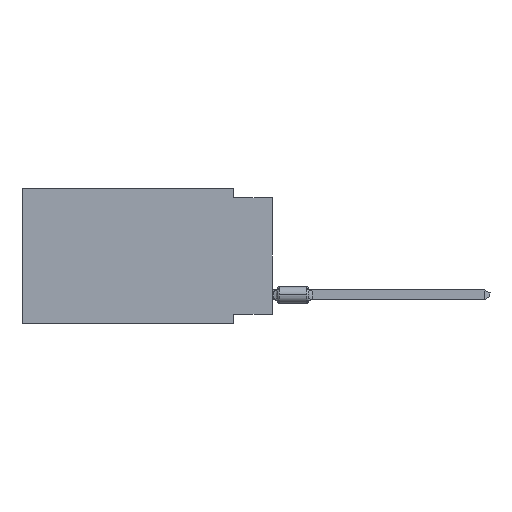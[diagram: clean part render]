
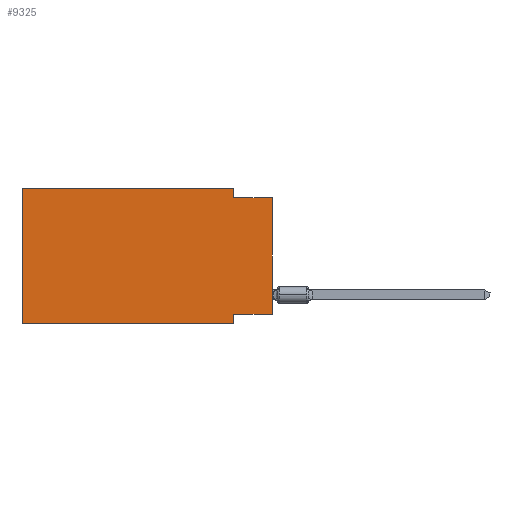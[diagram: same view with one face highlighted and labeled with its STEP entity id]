
A CAD part, left-side view. The second image highlights one B-rep face of the part: STEP entity #9325.
In plain terms, the highlighted planar face has unit normal (-1, 0, 0).
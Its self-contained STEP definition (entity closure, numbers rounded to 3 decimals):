
#4362 = CARTESIAN_POINT ( 'NONE',  ( 0., 0., -8.255 ) ) ;
#4892 = CARTESIAN_POINT ( 'NONE',  ( 0., 16.383, 0. ) ) ;
#5781 = LINE ( 'NONE', #65167, #79545 ) ;
#6080 = ORIENTED_EDGE ( 'NONE', *, *, #14157, .F. ) ;
#9325 = ADVANCED_FACE ( 'NONE', ( #74320 ), #50136, .F. ) ;
#11411 = VECTOR ( 'NONE', #47789, 1000. ) ;
#12465 = VERTEX_POINT ( 'NONE', #30352 ) ;
#12627 = ORIENTED_EDGE ( 'NONE', *, *, #22185, .T. ) ;
#14157 = EDGE_CURVE ( 'NONE', #34198, #68953, #107181, .T. ) ;
#14980 = AXIS2_PLACEMENT_3D ( 'NONE', #24831, #90823, #15455 ) ;
#15455 = DIRECTION ( 'NONE',  ( 0., 0., -1. ) ) ;
#17188 = VECTOR ( 'NONE', #23600, 1000. ) ;
#20465 = VERTEX_POINT ( 'NONE', #93433 ) ;
#20849 = LINE ( 'NONE', #4362, #53520 ) ;
#22127 = DIRECTION ( 'NONE',  ( 0., -1., 0. ) ) ;
#22185 = EDGE_CURVE ( 'NONE', #105822, #54163, #40701, .T. ) ;
#23600 = DIRECTION ( 'NONE',  ( 0., 0., -1. ) ) ;
#24831 = CARTESIAN_POINT ( 'NONE',  ( 0., 16.383, 0. ) ) ;
#26193 = ORIENTED_EDGE ( 'NONE', *, *, #58743, .F. ) ;
#26703 = CARTESIAN_POINT ( 'NONE',  ( 0., 2.54, -0.635 ) ) ;
#27291 = DIRECTION ( 'NONE',  ( 0., -1., 0. ) ) ;
#29407 = DIRECTION ( 'NONE',  ( 0., 0., -1. ) ) ;
#30352 = CARTESIAN_POINT ( 'NONE',  ( 0., 0., -8.255 ) ) ;
#31356 = VERTEX_POINT ( 'NONE', #39038 ) ;
#31867 = CARTESIAN_POINT ( 'NONE',  ( 0., 2.54, 0. ) ) ;
#32450 = CARTESIAN_POINT ( 'NONE',  ( 0., 2.54, -8.255 ) ) ;
#34198 = VERTEX_POINT ( 'NONE', #89519 ) ;
#35280 = VECTOR ( 'NONE', #22127, 1000. ) ;
#36018 = ORIENTED_EDGE ( 'NONE', *, *, #93101, .F. ) ;
#36579 = EDGE_LOOP ( 'NONE', ( #37124, #86515, #6080, #26193, #47039, #12627, #36018, #60204 ) ) ;
#36853 = VECTOR ( 'NONE', #38467, 1000. ) ;
#37124 = ORIENTED_EDGE ( 'NONE', *, *, #92950, .T. ) ;
#37690 = CARTESIAN_POINT ( 'NONE',  ( 0., 2.54, -8.89 ) ) ;
#38467 = DIRECTION ( 'NONE',  ( 0., -1., 0. ) ) ;
#39008 = LINE ( 'NONE', #91187, #11411 ) ;
#39038 = CARTESIAN_POINT ( 'NONE',  ( 0., 16.383, 0. ) ) ;
#40701 = LINE ( 'NONE', #58818, #58332 ) ;
#41904 = VERTEX_POINT ( 'NONE', #32450 ) ;
#47039 = ORIENTED_EDGE ( 'NONE', *, *, #67208, .F. ) ;
#47232 = VECTOR ( 'NONE', #29407, 1000. ) ;
#47789 = DIRECTION ( 'NONE',  ( 0., 0., 1. ) ) ;
#50136 = PLANE ( 'NONE',  #14980 ) ;
#53520 = VECTOR ( 'NONE', #71988, 1000. ) ;
#54163 = VERTEX_POINT ( 'NONE', #91049 ) ;
#58332 = VECTOR ( 'NONE', #27291, 1000. ) ;
#58743 = EDGE_CURVE ( 'NONE', #31356, #34198, #63758, .T. ) ;
#58818 = CARTESIAN_POINT ( 'NONE',  ( 0., 16.383, -8.89 ) ) ;
#60204 = ORIENTED_EDGE ( 'NONE', *, *, #68306, .F. ) ;
#63758 = LINE ( 'NONE', #4892, #36853 ) ;
#65167 = CARTESIAN_POINT ( 'NONE',  ( 0., 0., 0. ) ) ;
#65559 = LINE ( 'NONE', #97461, #35280 ) ;
#67208 = EDGE_CURVE ( 'NONE', #105822, #31356, #39008, .T. ) ;
#68306 = EDGE_CURVE ( 'NONE', #12465, #41904, #20849, .T. ) ;
#68953 = VERTEX_POINT ( 'NONE', #26703 ) ;
#71199 = LINE ( 'NONE', #37690, #47232 ) ;
#71988 = DIRECTION ( 'NONE',  ( 0., 1., 0. ) ) ;
#74320 = FACE_OUTER_BOUND ( 'NONE', #36579, .T. ) ;
#79545 = VECTOR ( 'NONE', #98677, 1000. ) ;
#86515 = ORIENTED_EDGE ( 'NONE', *, *, #99346, .F. ) ;
#88708 = CARTESIAN_POINT ( 'NONE',  ( 0., 16.383, -8.89 ) ) ;
#89519 = CARTESIAN_POINT ( 'NONE',  ( 0., 2.54, 0. ) ) ;
#90823 = DIRECTION ( 'NONE',  ( 1., 0., 0. ) ) ;
#91049 = CARTESIAN_POINT ( 'NONE',  ( 0., 2.54, -8.89 ) ) ;
#91187 = CARTESIAN_POINT ( 'NONE',  ( 0., 16.383, 0. ) ) ;
#92950 = EDGE_CURVE ( 'NONE', #12465, #20465, #5781, .T. ) ;
#93101 = EDGE_CURVE ( 'NONE', #41904, #54163, #71199, .T. ) ;
#93433 = CARTESIAN_POINT ( 'NONE',  ( 0., 0., -0.635 ) ) ;
#97461 = CARTESIAN_POINT ( 'NONE',  ( 0., 0., -0.635 ) ) ;
#98677 = DIRECTION ( 'NONE',  ( 0., 0., 1. ) ) ;
#99346 = EDGE_CURVE ( 'NONE', #68953, #20465, #65559, .T. ) ;
#105822 = VERTEX_POINT ( 'NONE', #88708 ) ;
#107181 = LINE ( 'NONE', #31867, #17188 ) ;
